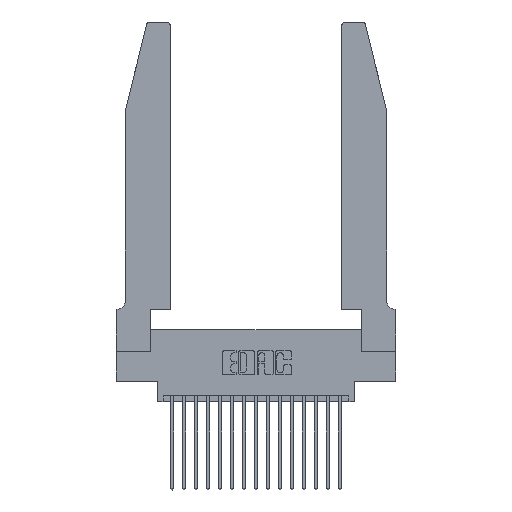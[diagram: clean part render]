
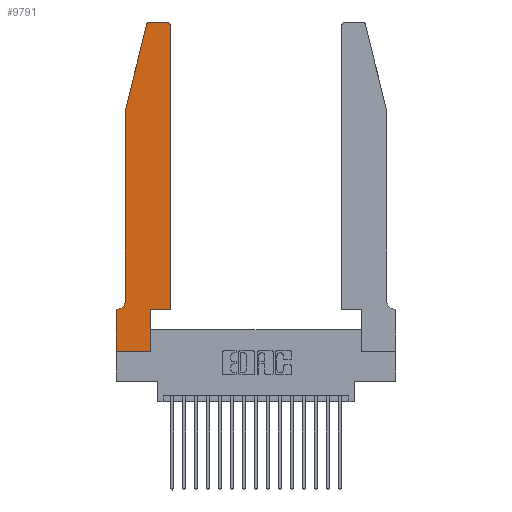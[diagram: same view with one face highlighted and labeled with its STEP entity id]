
A CAD part, top view. The second image highlights one B-rep face of the part: STEP entity #9791.
In plain terms, the highlighted planar face has unit normal (0, 0, 1).
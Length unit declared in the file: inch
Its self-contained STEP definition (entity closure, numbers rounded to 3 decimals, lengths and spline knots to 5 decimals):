
#16 = ORIENTED_EDGE ( 'NONE', *, *, #18762, .T. ) ;
#112 = CARTESIAN_POINT ( 'NONE',  ( 0., 0.35, 0.37 ) ) ;
#164 = AXIS2_PLACEMENT_3D ( 'NONE', #8965, #18147, #12000 ) ;
#340 = EDGE_CURVE ( 'NONE', #13804, #6825, #13837, .T. ) ;
#376 = CARTESIAN_POINT ( 'NONE',  ( 0., 0., 0.37 ) ) ;
#448 = CARTESIAN_POINT ( 'NONE',  ( 0.2865, 0.35, 0.37 ) ) ;
#485 = ORIENTED_EDGE ( 'NONE', *, *, #15024, .T. ) ;
#556 = CARTESIAN_POINT ( 'NONE',  ( 0.0755, 0.42, 0.37 ) ) ;
#841 = CARTESIAN_POINT ( 'NONE',  ( 0., 0.35, 0.37 ) ) ;
#1146 = LINE ( 'NONE', #15483, #4322 ) ;
#1184 = DIRECTION ( 'NONE',  ( 0., 0., -1. ) ) ;
#1245 = DIRECTION ( 'NONE',  ( 0., 1., 0. ) ) ;
#1286 = DIRECTION ( 'NONE',  ( -1., 0., 0. ) ) ;
#1951 = LINE ( 'NONE', #7210, #14001 ) ;
#2165 = EDGE_CURVE ( 'NONE', #11515, #3692, #20139, .T. ) ;
#2253 = CARTESIAN_POINT ( 'NONE',  ( 0.4205, 2.75, 0.37 ) ) ;
#2348 = VERTEX_POINT ( 'NONE', #14321 ) ;
#2663 = EDGE_CURVE ( 'NONE', #3712, #6513, #9572, .T. ) ;
#3256 = CARTESIAN_POINT ( 'NONE',  ( 0.284, 2.75, 0.37 ) ) ;
#3365 = EDGE_LOOP ( 'NONE', ( #5781, #20337, #12454, #14006, #16, #3756, #19322, #485, #18801, #15470, #11715, #7573 ) ) ;
#3487 = DIRECTION ( 'NONE',  ( 0., -1., 0. ) ) ;
#3549 = DIRECTION ( 'NONE',  ( 1., 0., 0. ) ) ;
#3692 = VERTEX_POINT ( 'NONE', #448 ) ;
#3712 = VERTEX_POINT ( 'NONE', #19032 ) ;
#3756 = ORIENTED_EDGE ( 'NONE', *, *, #10733, .T. ) ;
#3788 = VECTOR ( 'NONE', #3549, 39.37008 ) ;
#3793 = CARTESIAN_POINT ( 'NONE',  ( 0.4505, 0.35, 0.37 ) ) ;
#4272 = AXIS2_PLACEMENT_3D ( 'NONE', #19651, #10902, #11436 ) ;
#4322 = VECTOR ( 'NONE', #1286, 39.37008 ) ;
#4660 = LINE ( 'NONE', #9691, #8853 ) ;
#5207 = CARTESIAN_POINT ( 'NONE',  ( 0.0755, 2., 0.37 ) ) ;
#5781 = ORIENTED_EDGE ( 'NONE', *, *, #17856, .T. ) ;
#6509 = LINE ( 'NONE', #376, #3788 ) ;
#6513 = VERTEX_POINT ( 'NONE', #2253 ) ;
#6554 = EDGE_CURVE ( 'NONE', #2348, #3712, #12152, .T. ) ;
#6595 = CARTESIAN_POINT ( 'NONE',  ( 0.25487, 2.72718, 0.37 ) ) ;
#6825 = VERTEX_POINT ( 'NONE', #6595 ) ;
#6840 = DIRECTION ( 'NONE',  ( 1., 0., 0. ) ) ;
#6915 = EDGE_CURVE ( 'NONE', #14289, #13982, #6970, .T. ) ;
#6970 = LINE ( 'NONE', #5207, #15539 ) ;
#7210 = CARTESIAN_POINT ( 'NONE',  ( 0.2605, 2.75, 0.37 ) ) ;
#7491 = DIRECTION ( 'NONE',  ( -1., 0., 0. ) ) ;
#7573 = ORIENTED_EDGE ( 'NONE', *, *, #2663, .T. ) ;
#8440 = VECTOR ( 'NONE', #1245, 39.37008 ) ;
#8634 = CARTESIAN_POINT ( 'NONE',  ( 0.2865, 0.35, 0.37 ) ) ;
#8835 = DIRECTION ( 'NONE',  ( 0., 1., 0. ) ) ;
#8853 = VECTOR ( 'NONE', #11069, 39.37008 ) ;
#8854 = EDGE_CURVE ( 'NONE', #6825, #14289, #12045, .T. ) ;
#8965 = CARTESIAN_POINT ( 'NONE',  ( 0.284, 2.72, 0.37 ) ) ;
#9572 = CIRCLE ( 'NONE', #4272, 0.03 ) ;
#9691 = CARTESIAN_POINT ( 'NONE',  ( 0., 0., 0.37 ) ) ;
#9773 = FACE_OUTER_BOUND ( 'NONE', #3365, .T. ) ;
#9791 = ADVANCED_FACE ( 'NONE', ( #9773 ), #11510, .T. ) ;
#10401 = DIRECTION ( 'NONE',  ( 1., 0., 0. ) ) ;
#10733 = EDGE_CURVE ( 'NONE', #13930, #18318, #1146, .T. ) ;
#10902 = DIRECTION ( 'NONE',  ( 0., 0., 1. ) ) ;
#11069 = DIRECTION ( 'NONE',  ( 0., -1., 0. ) ) ;
#11436 = DIRECTION ( 'NONE',  ( 1., 0., 0. ) ) ;
#11510 = PLANE ( 'NONE',  #17523 ) ;
#11515 = VERTEX_POINT ( 'NONE', #17462 ) ;
#11715 = ORIENTED_EDGE ( 'NONE', *, *, #6554, .T. ) ;
#12000 = DIRECTION ( 'NONE',  ( 1., 0., 0. ) ) ;
#12045 = LINE ( 'NONE', #14840, #13994 ) ;
#12152 = LINE ( 'NONE', #15038, #8440 ) ;
#12235 = LINE ( 'NONE', #3793, #15385 ) ;
#12420 = AXIS2_PLACEMENT_3D ( 'NONE', #15303, #1184, #7491 ) ;
#12454 = ORIENTED_EDGE ( 'NONE', *, *, #8854, .T. ) ;
#12523 = CIRCLE ( 'NONE', #12420, 0.07 ) ;
#13160 = DIRECTION ( 'NONE',  ( -0.239, -0.971, 0. ) ) ;
#13299 = CARTESIAN_POINT ( 'NONE',  ( 0.0055, 0.35, 0.37 ) ) ;
#13804 = VERTEX_POINT ( 'NONE', #3256 ) ;
#13837 = CIRCLE ( 'NONE', #164, 0.03 ) ;
#13930 = VERTEX_POINT ( 'NONE', #13299 ) ;
#13982 = VERTEX_POINT ( 'NONE', #556 ) ;
#13994 = VECTOR ( 'NONE', #13160, 39.37008 ) ;
#14001 = VECTOR ( 'NONE', #19556, 39.37008 ) ;
#14006 = ORIENTED_EDGE ( 'NONE', *, *, #6915, .T. ) ;
#14289 = VERTEX_POINT ( 'NONE', #17247 ) ;
#14321 = CARTESIAN_POINT ( 'NONE',  ( 0.4505, 0.35, 0.37 ) ) ;
#14840 = CARTESIAN_POINT ( 'NONE',  ( 0.0755, 2., 0.37 ) ) ;
#14980 = VECTOR ( 'NONE', #8835, 39.37008 ) ;
#15024 = EDGE_CURVE ( 'NONE', #16430, #11515, #6509, .T. ) ;
#15038 = CARTESIAN_POINT ( 'NONE',  ( 0.4505, 0.35, 0.37 ) ) ;
#15303 = CARTESIAN_POINT ( 'NONE',  ( 0.0055, 0.42, 0.37 ) ) ;
#15385 = VECTOR ( 'NONE', #6840, 39.37008 ) ;
#15470 = ORIENTED_EDGE ( 'NONE', *, *, #19637, .T. ) ;
#15483 = CARTESIAN_POINT ( 'NONE',  ( 0.0755, 0.35, 0.37 ) ) ;
#15539 = VECTOR ( 'NONE', #3487, 39.37008 ) ;
#15759 = CARTESIAN_POINT ( 'NONE',  ( 0., 0., 0.37 ) ) ;
#16430 = VERTEX_POINT ( 'NONE', #15759 ) ;
#17247 = CARTESIAN_POINT ( 'NONE',  ( 0.0755, 2., 0.37 ) ) ;
#17462 = CARTESIAN_POINT ( 'NONE',  ( 0.2865, 0., 0.37 ) ) ;
#17523 = AXIS2_PLACEMENT_3D ( 'NONE', #841, #19786, #10401 ) ;
#17652 = EDGE_CURVE ( 'NONE', #18318, #16430, #4660, .T. ) ;
#17856 = EDGE_CURVE ( 'NONE', #6513, #13804, #1951, .T. ) ;
#18147 = DIRECTION ( 'NONE',  ( 0., 0., 1. ) ) ;
#18318 = VERTEX_POINT ( 'NONE', #112 ) ;
#18762 = EDGE_CURVE ( 'NONE', #13982, #13930, #12523, .T. ) ;
#18801 = ORIENTED_EDGE ( 'NONE', *, *, #2165, .T. ) ;
#19032 = CARTESIAN_POINT ( 'NONE',  ( 0.4505, 2.72, 0.37 ) ) ;
#19322 = ORIENTED_EDGE ( 'NONE', *, *, #17652, .T. ) ;
#19556 = DIRECTION ( 'NONE',  ( -1., 0., 0. ) ) ;
#19637 = EDGE_CURVE ( 'NONE', #3692, #2348, #12235, .T. ) ;
#19651 = CARTESIAN_POINT ( 'NONE',  ( 0.4205, 2.72, 0.37 ) ) ;
#19786 = DIRECTION ( 'NONE',  ( 0., 0., 1. ) ) ;
#20139 = LINE ( 'NONE', #8634, #14980 ) ;
#20337 = ORIENTED_EDGE ( 'NONE', *, *, #340, .T. ) ;
